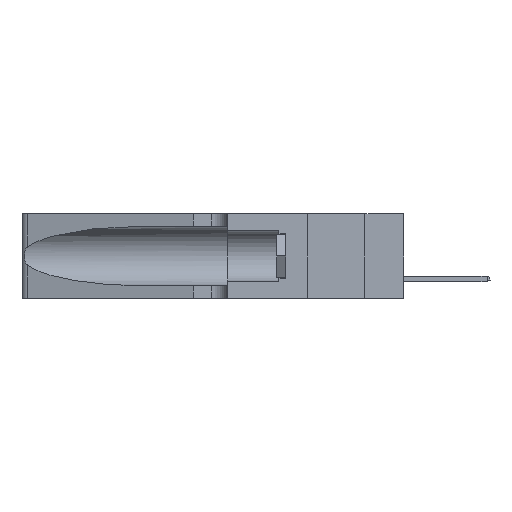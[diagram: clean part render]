
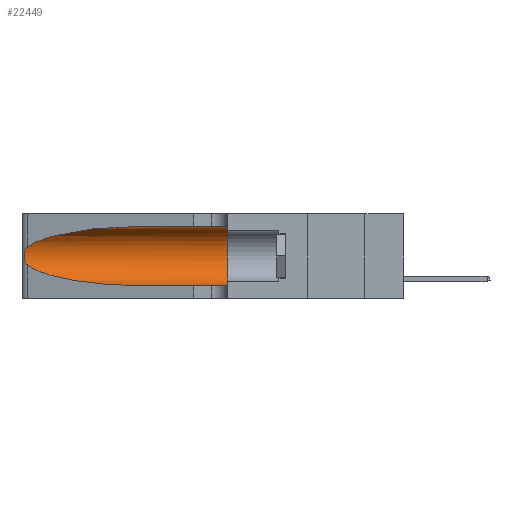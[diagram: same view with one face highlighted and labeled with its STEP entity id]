
A CAD part, left-side view. The second image highlights one B-rep face of the part: STEP entity #22449.
In plain terms, the highlighted cylindrical face has radius 3.308 mm (diameter 6.617 mm), a partial arc.
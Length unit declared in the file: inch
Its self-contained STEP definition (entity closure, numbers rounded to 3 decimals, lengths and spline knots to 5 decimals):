
#296 = CARTESIAN_POINT ( 'NONE',  ( 0.25639, 1.23184, 0.21858 ) ) ;
#821 = DIRECTION ( 'NONE',  ( 0., -1., 0. ) ) ;
#2030 = ORIENTED_EDGE ( 'NONE', *, *, #41832, .T. ) ;
#2279 = FACE_OUTER_BOUND ( 'NONE', #25812, .T. ) ;
#2785 = CARTESIAN_POINT ( 'NONE',  ( 0.1305, 1.61858, 0.31525 ) ) ;
#3362 = CARTESIAN_POINT ( 'NONE',  ( 0.1305, 1.61858, 0.185 ) ) ;
#3583 = CARTESIAN_POINT ( 'NONE',  ( 0.25487, 1.22718, 0.14631 ) ) ;
#3797 = VERTEX_POINT ( 'NONE', #11825 ) ;
#3958 = CARTESIAN_POINT ( 'NONE',  ( 0.1305, 0.35, 0.185 ) ) ;
#5013 = VERTEX_POINT ( 'NONE', #20614 ) ;
#6451 = CARTESIAN_POINT ( 'NONE',  ( 0.25487, 1.22718, 0.14631 ) ) ;
#7074 = DIRECTION ( 'NONE',  ( 0., -1., 0. ) ) ;
#7694 = EDGE_CURVE ( 'NONE', #5013, #16121, #28343, .T. ) ;
#8874 = CARTESIAN_POINT ( 'NONE',  ( 0.1305, 0.35, 0.05475 ) ) ;
#9524 = ORIENTED_EDGE ( 'NONE', *, *, #36573, .F. ) ;
#10816 = CARTESIAN_POINT ( 'NONE',  ( 0.1305, 1.61858, 0.05475 ) ) ;
#11007 = CARTESIAN_POINT ( 'NONE',  ( 0.25787, 1.23484, 0.2124 ) ) ;
#11066 = DIRECTION ( 'NONE',  ( 0., 0., 1. ) ) ;
#11407 = DIRECTION ( 'NONE',  ( 0., 0., -1. ) ) ;
#11479 = CARTESIAN_POINT ( 'NONE',  ( 0.26075, 1.23896, 0.19203 ) ) ;
#11825 = CARTESIAN_POINT ( 'NONE',  ( 0.1305, 0.35, 0.31525 ) ) ;
#11987 = CARTESIAN_POINT ( 'NONE',  ( 0.25487, 1.22718, 0.14631 ) ) ;
#14124 = EDGE_CURVE ( 'NONE', #42475, #22862, #38826, .T. ) ;
#16121 = VERTEX_POINT ( 'NONE', #39828 ) ;
#16655 = EDGE_CURVE ( 'NONE', #5013, #3797, #28707, .T. ) ;
#17229 = ORIENTED_EDGE ( 'NONE', *, *, #7694, .T. ) ;
#18338 = CARTESIAN_POINT ( 'NONE',  ( 0.25789, 1.23486, 0.15765 ) ) ;
#18715 = DIRECTION ( 'NONE',  ( 0., 1., 0. ) ) ;
#19538 = CARTESIAN_POINT ( 'NONE',  ( 0.25487, 1.22718, 0.22369 ) ) ;
#20333 = AXIS2_PLACEMENT_3D ( 'NONE', #3362, #7074, #11407 ) ;
#20614 = CARTESIAN_POINT ( 'NONE',  ( 0.1305, 0.72297, 0.31525 ) ) ;
#21907 = CARTESIAN_POINT ( 'NONE',  ( 0.26018, 1.23835, 0.19895 ) ) ;
#22062 = CARTESIAN_POINT ( 'NONE',  ( 0.25555, 1.22993, 0.14849 ) ) ;
#22449 = ADVANCED_FACE ( 'NONE', ( #2279 ), #42315, .F. ) ;
#22862 = VERTEX_POINT ( 'NONE', #8874 ) ;
#23779 = VERTEX_POINT ( 'NONE', #11987 ) ;
#25680 = CARTESIAN_POINT ( 'NONE',  ( 0.26017, 1.23833, 0.17102 ) ) ;
#25812 = EDGE_LOOP ( 'NONE', ( #17229, #2030, #45479, #27210, #9524, #33580 ) ) ;
#26169 = CARTESIAN_POINT ( 'NONE',  ( 0.1305, 0.72297, 0.05475 ) ) ;
#27130 = EDGE_CURVE ( 'NONE', #23779, #42475, #47681, .T. ) ;
#27210 = ORIENTED_EDGE ( 'NONE', *, *, #14124, .T. ) ;
#27331 = AXIS2_PLACEMENT_3D ( 'NONE', #3958, #18715, #11066 ) ;
#27534 = VECTOR ( 'NONE', #821, 39.37008 ) ;
#28343 =( BOUNDED_CURVE ( )  B_SPLINE_CURVE ( 3, ( #44531, #33501, #34333, #19538 ),
 .UNSPECIFIED., .F., .F. ) 
 B_SPLINE_CURVE_WITH_KNOTS ( ( 4, 4 ),
 ( 1.5708, 2.84003 ),
 .UNSPECIFIED. ) 
 CURVE ( )  GEOMETRIC_REPRESENTATION_ITEM ( )  RATIONAL_B_SPLINE_CURVE ( ( 1., 0.87, 0.87, 1. ) ) 
 REPRESENTATION_ITEM ( '' )  );
#28707 = LINE ( 'NONE', #2785, #27534 ) ;
#29821 = DIRECTION ( 'NONE',  ( 0., -1., 0. ) ) ;
#30036 = CARTESIAN_POINT ( 'NONE',  ( 0.25555, 1.22994, 0.2215 ) ) ;
#31801 = CARTESIAN_POINT ( 'NONE',  ( 0.2373, 1.15595, 0.08982 ) ) ;
#31854 = VECTOR ( 'NONE', #29821, 39.37008 ) ;
#33276 = CARTESIAN_POINT ( 'NONE',  ( 0.25854, 1.2359, 0.20912 ) ) ;
#33501 = CARTESIAN_POINT ( 'NONE',  ( 0.18966, 0.96281, 0.31525 ) ) ;
#33580 = ORIENTED_EDGE ( 'NONE', *, *, #16655, .F. ) ;
#34333 = CARTESIAN_POINT ( 'NONE',  ( 0.2373, 1.15595, 0.28018 ) ) ;
#35560 = CARTESIAN_POINT ( 'NONE',  ( 0.18966, 0.96281, 0.05475 ) ) ;
#36573 = EDGE_CURVE ( 'NONE', #3797, #22862, #45585, .T. ) ;
#36874 = CARTESIAN_POINT ( 'NONE',  ( 0.25856, 1.23593, 0.16098 ) ) ;
#37957 = CARTESIAN_POINT ( 'NONE',  ( 0.1305, 0.72297, 0.05475 ) ) ;
#38826 = LINE ( 'NONE', #10816, #31854 ) ;
#39828 = CARTESIAN_POINT ( 'NONE',  ( 0.25487, 1.22718, 0.22369 ) ) ;
#41071 = CARTESIAN_POINT ( 'NONE',  ( 0.25487, 1.22718, 0.22369 ) ) ;
#41832 = EDGE_CURVE ( 'NONE', #16121, #23779, #46483, .T. ) ;
#42315 = CYLINDRICAL_SURFACE ( 'NONE', #20333, 0.13025 ) ;
#42475 = VERTEX_POINT ( 'NONE', #37957 ) ;
#44314 = CARTESIAN_POINT ( 'NONE',  ( 0.25639, 1.23186, 0.15144 ) ) ;
#44531 = CARTESIAN_POINT ( 'NONE',  ( 0.1305, 0.72297, 0.31525 ) ) ;
#45479 = ORIENTED_EDGE ( 'NONE', *, *, #27130, .T. ) ;
#45585 = CIRCLE ( 'NONE', #27331, 0.13025 ) ;
#46483 = B_SPLINE_CURVE_WITH_KNOTS ( 'NONE', 3,
 ( #41071, #30036, #296, #11007, #33276, #21907, #11479, #47906, #25680, #36874, #18338, #44314, #22062, #3583 ),
 .UNSPECIFIED., .F., .F.,
 ( 4, 2, 2, 2, 2, 2, 4 ),
 ( 0., 0.00027, 0.00053, 0.00107, 0.0016, 0.00187, 0.00214 ),
 .UNSPECIFIED. ) ;
#47681 =( BOUNDED_CURVE ( )  B_SPLINE_CURVE ( 3, ( #6451, #31801, #35560, #26169 ),
 .UNSPECIFIED., .F., .F. ) 
 B_SPLINE_CURVE_WITH_KNOTS ( ( 4, 4 ),
 ( 3.44316, 4.71239 ),
 .UNSPECIFIED. ) 
 CURVE ( )  GEOMETRIC_REPRESENTATION_ITEM ( )  RATIONAL_B_SPLINE_CURVE ( ( 1., 0.87, 0.87, 1. ) ) 
 REPRESENTATION_ITEM ( '' )  );
#47906 = CARTESIAN_POINT ( 'NONE',  ( 0.26075, 1.23896, 0.178 ) ) ;
